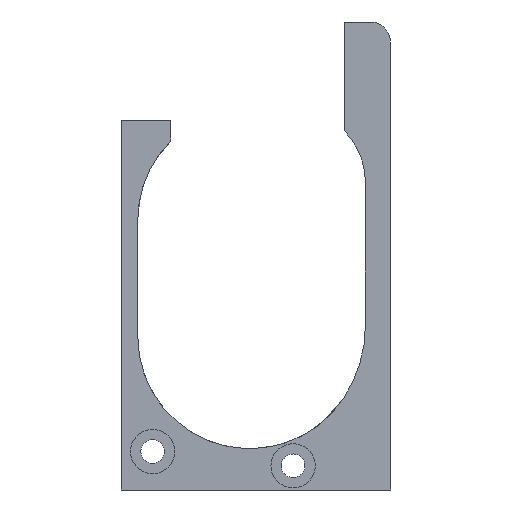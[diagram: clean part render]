
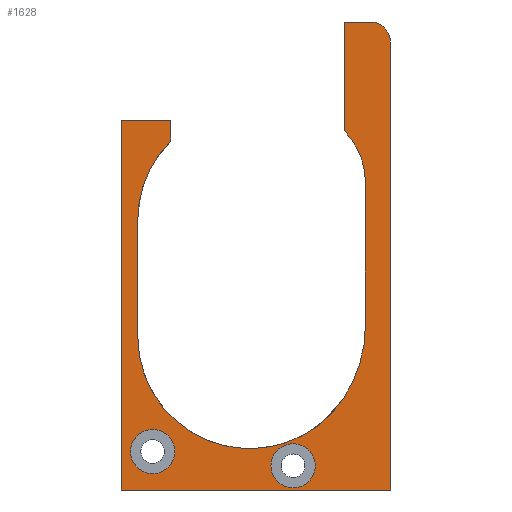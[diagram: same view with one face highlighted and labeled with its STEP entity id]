
A CAD part, left-side view. The second image highlights one B-rep face of the part: STEP entity #1628.
In plain terms, the highlighted planar face has unit normal (-1, 0, 0).
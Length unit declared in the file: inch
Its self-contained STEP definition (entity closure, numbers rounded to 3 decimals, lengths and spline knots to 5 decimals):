
#16=FACE_BOUND('',#243,.T.);
#17=FACE_BOUND('',#244,.T.);
#29=PLANE('',#1717);
#68=CIRCLE('',#1718,0.1);
#69=CIRCLE('',#1719,0.37093);
#70=CIRCLE('',#1720,0.66145);
#71=CIRCLE('',#1721,0.559);
#72=CIRCLE('',#1722,0.559);
#73=CIRCLE('',#1723,0.11024);
#74=CIRCLE('',#1724,0.11024);
#152=FACE_OUTER_BOUND('',#242,.T.);
#242=EDGE_LOOP('',(#1285,#1286,#1287,#1288,#1289,#1290,#1291,#1292,#1293,
#1294,#1295,#1296,#1297,#1298));
#243=EDGE_LOOP('',(#1299));
#244=EDGE_LOOP('',(#1300));
#456=LINE('',#4700,#532);
#459=LINE('',#4778,#535);
#461=LINE('',#4782,#537);
#462=LINE('',#4784,#538);
#463=LINE('',#4786,#539);
#464=LINE('',#4790,#540);
#465=LINE('',#4792,#541);
#466=LINE('',#4796,#542);
#467=LINE('',#4802,#543);
#532=VECTOR('',#1866,0.3937);
#535=VECTOR('',#1889,0.3937);
#537=VECTOR('',#1893,0.3937);
#538=VECTOR('',#1894,0.3937);
#539=VECTOR('',#1895,0.3937);
#540=VECTOR('',#1898,0.3937);
#541=VECTOR('',#1899,0.3937);
#542=VECTOR('',#1902,0.3937);
#543=VECTOR('',#1907,0.3937);
#701=VERTEX_POINT('',#4697);
#702=VERTEX_POINT('',#4699);
#705=VERTEX_POINT('',#4777);
#706=VERTEX_POINT('',#4781);
#707=VERTEX_POINT('',#4783);
#708=VERTEX_POINT('',#4785);
#709=VERTEX_POINT('',#4787);
#710=VERTEX_POINT('',#4789);
#711=VERTEX_POINT('',#4791);
#712=VERTEX_POINT('',#4793);
#713=VERTEX_POINT('',#4795);
#714=VERTEX_POINT('',#4797);
#715=VERTEX_POINT('',#4799);
#716=VERTEX_POINT('',#4801);
#717=VERTEX_POINT('',#4804);
#718=VERTEX_POINT('',#4806);
#912=EDGE_CURVE('',#701,#702,#456,.T.);
#931=EDGE_CURVE('',#702,#705,#459,.T.);
#933=EDGE_CURVE('',#701,#706,#461,.T.);
#934=EDGE_CURVE('',#707,#706,#462,.T.);
#935=EDGE_CURVE('',#708,#707,#463,.T.);
#936=EDGE_CURVE('',#709,#708,#68,.T.);
#937=EDGE_CURVE('',#710,#709,#464,.T.);
#938=EDGE_CURVE('',#710,#711,#465,.F.);
#939=EDGE_CURVE('',#712,#711,#69,.T.);
#940=EDGE_CURVE('',#713,#712,#466,.T.);
#941=EDGE_CURVE('',#714,#713,#70,.T.);
#942=EDGE_CURVE('',#715,#714,#71,.T.);
#943=EDGE_CURVE('',#715,#716,#467,.T.);
#944=EDGE_CURVE('',#705,#716,#72,.T.);
#945=EDGE_CURVE('',#717,#717,#73,.T.);
#946=EDGE_CURVE('',#718,#718,#74,.T.);
#1285=ORIENTED_EDGE('',*,*,#931,.F.);
#1286=ORIENTED_EDGE('',*,*,#912,.F.);
#1287=ORIENTED_EDGE('',*,*,#933,.T.);
#1288=ORIENTED_EDGE('',*,*,#934,.F.);
#1289=ORIENTED_EDGE('',*,*,#935,.F.);
#1290=ORIENTED_EDGE('',*,*,#936,.F.);
#1291=ORIENTED_EDGE('',*,*,#937,.F.);
#1292=ORIENTED_EDGE('',*,*,#938,.T.);
#1293=ORIENTED_EDGE('',*,*,#939,.F.);
#1294=ORIENTED_EDGE('',*,*,#940,.F.);
#1295=ORIENTED_EDGE('',*,*,#941,.F.);
#1296=ORIENTED_EDGE('',*,*,#942,.F.);
#1297=ORIENTED_EDGE('',*,*,#943,.T.);
#1298=ORIENTED_EDGE('',*,*,#944,.F.);
#1299=ORIENTED_EDGE('',*,*,#945,.T.);
#1300=ORIENTED_EDGE('',*,*,#946,.T.);
#1628=ADVANCED_FACE('',(#152,#16,#17),#29,.F.);
#1717=AXIS2_PLACEMENT_3D('',#4780,#1891,#1892);
#1718=AXIS2_PLACEMENT_3D('',#4788,#1896,#1897);
#1719=AXIS2_PLACEMENT_3D('',#4794,#1900,#1901);
#1720=AXIS2_PLACEMENT_3D('',#4798,#1903,#1904);
#1721=AXIS2_PLACEMENT_3D('',#4800,#1905,#1906);
#1722=AXIS2_PLACEMENT_3D('',#4803,#1908,#1909);
#1723=AXIS2_PLACEMENT_3D('',#4805,#1910,#1911);
#1724=AXIS2_PLACEMENT_3D('',#4807,#1912,#1913);
#1866=DIRECTION('',(0.,-1.,0.));
#1889=DIRECTION('',(0.,0.,-1.));
#1891=DIRECTION('center_axis',(1.,0.,0.));
#1892=DIRECTION('ref_axis',(0.,0.,-1.));
#1893=DIRECTION('',(0.,0.,-1.));
#1894=DIRECTION('',(0.,1.,0.));
#1895=DIRECTION('',(0.,0.,-1.));
#1896=DIRECTION('center_axis',(1.,0.,0.));
#1897=DIRECTION('ref_axis',(0.,-0.707,0.707));
#1898=DIRECTION('',(0.,-1.,0.));
#1899=DIRECTION('',(0.,0.,1.));
#1900=DIRECTION('center_axis',(-1.,0.,0.));
#1901=DIRECTION('ref_axis',(0.,-1.,0.));
#1902=DIRECTION('',(0.,0.,1.));
#1903=DIRECTION('center_axis',(-1.,0.,0.));
#1904=DIRECTION('ref_axis',(0.,-0.834,-0.552));
#1905=DIRECTION('center_axis',(-1.,0.,0.));
#1906=DIRECTION('ref_axis',(0.,0.,1.));
#1907=DIRECTION('',(0.,0.,1.));
#1908=DIRECTION('center_axis',(-1.,0.,0.));
#1909=DIRECTION('ref_axis',(0.,0.707,0.707));
#1910=DIRECTION('center_axis',(1.,0.,0.));
#1911=DIRECTION('ref_axis',(0.,0.,1.));
#1912=DIRECTION('center_axis',(1.,0.,0.));
#1913=DIRECTION('ref_axis',(0.,0.,1.));
#4697=CARTESIAN_POINT('',(-0.363,-1.254,-0.095));
#4699=CARTESIAN_POINT('',(-0.363,-1.49873,-0.095));
#4700=CARTESIAN_POINT('',(-0.363,-1.14261,-0.095));
#4777=CARTESIAN_POINT('',(-0.363,-1.49873,-0.19873));
#4778=CARTESIAN_POINT('',(-0.363,-1.49873,-1.10811));
#4780=CARTESIAN_POINT('Origin',(-0.363,-0.7865,-2.0175));
#4781=CARTESIAN_POINT('',(-0.363,-1.254,-1.938));
#4782=CARTESIAN_POINT('',(-0.363,-1.254,-1.72625));
#4783=CARTESIAN_POINT('',(-0.363,-2.595,-1.938));
#4784=CARTESIAN_POINT('',(-0.363,-1.01361,-1.938));
#4785=CARTESIAN_POINT('',(-0.363,-2.595,0.295));
#4786=CARTESIAN_POINT('',(-0.363,-2.595,-1.41725));
#4787=CARTESIAN_POINT('',(-0.363,-2.495,0.395));
#4788=CARTESIAN_POINT('Origin',(-0.363,-2.495,0.295));
#4789=CARTESIAN_POINT('',(-0.363,-2.36436,0.395));
#4790=CARTESIAN_POINT('',(-0.363,-2.28,0.395));
#4791=CARTESIAN_POINT('',(-0.363,-2.36436,-0.14668));
#4792=CARTESIAN_POINT('',(-0.363,-2.36436,-1.08057));
#4793=CARTESIAN_POINT('',(-0.363,-2.47,-0.40593));
#4794=CARTESIAN_POINT('Origin',(-0.363,-2.09907,-0.40593));
#4795=CARTESIAN_POINT('',(-0.363,-2.47,-1.11648));
#4796=CARTESIAN_POINT('',(-0.363,-2.47,-0.65121));
#4797=CARTESIAN_POINT('',(-0.363,-2.36024,-1.48138));
#4798=CARTESIAN_POINT('Origin',(-0.363,-1.80855,-1.11648));
#4799=CARTESIAN_POINT('',(-0.363,-1.335,-1.173));
#4800=CARTESIAN_POINT('Origin',(-0.363,-1.894,-1.173));
#4801=CARTESIAN_POINT('',(-0.363,-1.335,-0.594));
#4802=CARTESIAN_POINT('',(-0.363,-1.335,-1.00875));
#4803=CARTESIAN_POINT('Origin',(-0.363,-1.894,-0.594));
#4804=CARTESIAN_POINT('',(-0.363,-2.1095,-1.9277));
#4805=CARTESIAN_POINT('Origin',(-0.363,-2.1095,-1.81746));
#4806=CARTESIAN_POINT('',(-0.363,-1.4095,-1.85659));
#4807=CARTESIAN_POINT('Origin',(-0.363,-1.4095,-1.74635));
